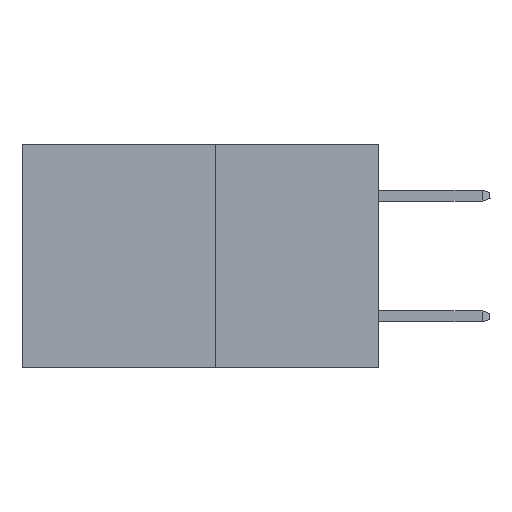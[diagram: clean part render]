
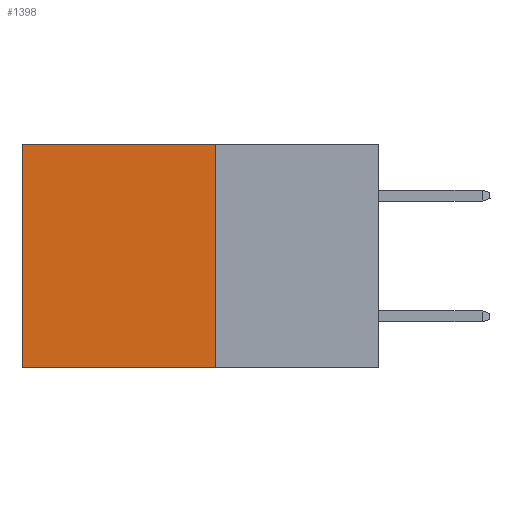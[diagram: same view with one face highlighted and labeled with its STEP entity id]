
A CAD part, left-side view. The second image highlights one B-rep face of the part: STEP entity #1398.
In plain terms, the highlighted planar face has unit normal (-1, 0, 0).
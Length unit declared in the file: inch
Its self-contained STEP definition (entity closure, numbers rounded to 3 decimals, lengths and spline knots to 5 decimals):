
#301 = EDGE_CURVE ( 'NONE', #6313, #6881, #3797, .T. ) ;
#359 = DIRECTION ( 'NONE',  ( 0., 1., 0. ) ) ;
#431 = CARTESIAN_POINT ( 'NONE',  ( 0.277, 0.59, -0.37 ) ) ;
#635 = ORIENTED_EDGE ( 'NONE', *, *, #3802, .T. ) ;
#793 = AXIS2_PLACEMENT_3D ( 'NONE', #3494, #6779, #5734 ) ;
#841 = VERTEX_POINT ( 'NONE', #7812 ) ;
#1211 = FACE_OUTER_BOUND ( 'NONE', #7247, .T. ) ;
#1257 = EDGE_CURVE ( 'NONE', #841, #6313, #5074, .T. ) ;
#1398 = ADVANCED_FACE ( 'NONE', ( #1211 ), #7353, .F. ) ;
#1525 = VECTOR ( 'NONE', #2387, 39.37008 ) ;
#1697 = VECTOR ( 'NONE', #7948, 39.37008 ) ;
#2387 = DIRECTION ( 'NONE',  ( 0., 1., 0. ) ) ;
#2465 = ORIENTED_EDGE ( 'NONE', *, *, #1257, .F. ) ;
#3037 = EDGE_CURVE ( 'NONE', #841, #6618, #3527, .T. ) ;
#3236 = CARTESIAN_POINT ( 'NONE',  ( 0.277, 0.27, 0. ) ) ;
#3260 = CARTESIAN_POINT ( 'NONE',  ( 0.277, 0.59, 0. ) ) ;
#3494 = CARTESIAN_POINT ( 'NONE',  ( 0.277, 0.27, -0.37 ) ) ;
#3527 = LINE ( 'NONE', #3236, #1525 ) ;
#3786 = CARTESIAN_POINT ( 'NONE',  ( 0.277, 0.27, -0.37 ) ) ;
#3797 = LINE ( 'NONE', #5577, #5573 ) ;
#3802 = EDGE_CURVE ( 'NONE', #6618, #6881, #5775, .T. ) ;
#4016 = VECTOR ( 'NONE', #6088, 39.37008 ) ;
#4173 = CARTESIAN_POINT ( 'NONE',  ( 0.277, 0.27, -0.37 ) ) ;
#4497 = ORIENTED_EDGE ( 'NONE', *, *, #301, .F. ) ;
#5074 = LINE ( 'NONE', #4173, #1697 ) ;
#5573 = VECTOR ( 'NONE', #359, 39.37008 ) ;
#5577 = CARTESIAN_POINT ( 'NONE',  ( 0.277, 0.27, -0.37 ) ) ;
#5734 = DIRECTION ( 'NONE',  ( 0., 0., -1. ) ) ;
#5775 = LINE ( 'NONE', #7227, #4016 ) ;
#6088 = DIRECTION ( 'NONE',  ( 0., 0., -1. ) ) ;
#6313 = VERTEX_POINT ( 'NONE', #3786 ) ;
#6618 = VERTEX_POINT ( 'NONE', #3260 ) ;
#6779 = DIRECTION ( 'NONE',  ( 1., 0., 0. ) ) ;
#6881 = VERTEX_POINT ( 'NONE', #431 ) ;
#7227 = CARTESIAN_POINT ( 'NONE',  ( 0.277, 0.59, -0.37 ) ) ;
#7247 = EDGE_LOOP ( 'NONE', ( #635, #4497, #2465, #7806 ) ) ;
#7353 = PLANE ( 'NONE',  #793 ) ;
#7806 = ORIENTED_EDGE ( 'NONE', *, *, #3037, .T. ) ;
#7812 = CARTESIAN_POINT ( 'NONE',  ( 0.277, 0.27, 0. ) ) ;
#7948 = DIRECTION ( 'NONE',  ( 0., 0., -1. ) ) ;
